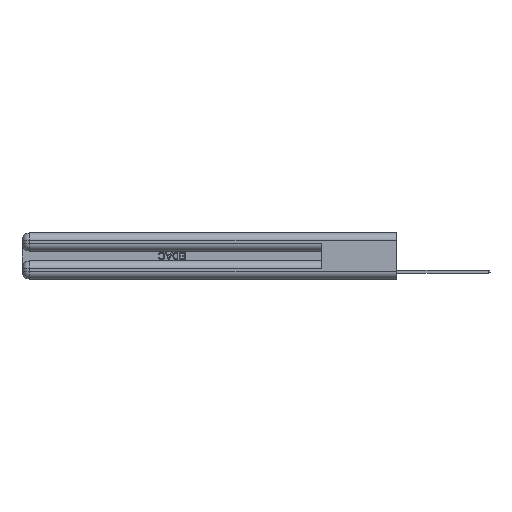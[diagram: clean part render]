
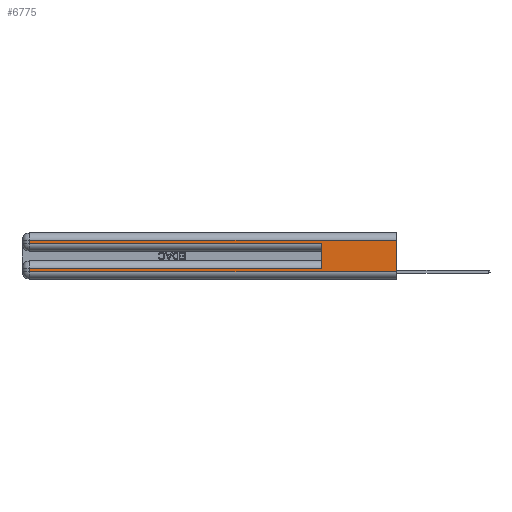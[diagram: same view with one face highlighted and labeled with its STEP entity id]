
A CAD part, left-side view. The second image highlights one B-rep face of the part: STEP entity #6775.
In plain terms, the highlighted planar face has unit normal (-1, 0, 0).
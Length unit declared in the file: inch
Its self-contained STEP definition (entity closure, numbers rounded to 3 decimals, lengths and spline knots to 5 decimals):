
#906 = EDGE_CURVE ( 'NONE', #27352, #23586, #1004, .T. ) ;
#1004 = LINE ( 'NONE', #22180, #7337 ) ;
#1892 = CARTESIAN_POINT ( 'NONE',  ( 0., 0.6, 0.085 ) ) ;
#3606 = VERTEX_POINT ( 'NONE', #33689 ) ;
#3704 = DIRECTION ( 'NONE',  ( 0., 0., 1. ) ) ;
#4698 = LINE ( 'NONE', #28986, #30235 ) ;
#5612 = DIRECTION ( 'NONE',  ( 0., 1., 0. ) ) ;
#5818 = CARTESIAN_POINT ( 'NONE',  ( 0., 0., 0.085 ) ) ;
#6775 = ADVANCED_FACE ( 'NONE', ( #32164 ), #9084, .F. ) ;
#7131 = EDGE_CURVE ( 'NONE', #3606, #16999, #32991, .T. ) ;
#7337 = VECTOR ( 'NONE', #27088, 39.37008 ) ;
#7918 = LINE ( 'NONE', #5818, #17480 ) ;
#9084 = PLANE ( 'NONE',  #31050 ) ;
#11957 = DIRECTION ( 'NONE',  ( 1., 0., 0. ) ) ;
#12300 = EDGE_CURVE ( 'NONE', #30285, #13682, #31809, .T. ) ;
#13682 = VERTEX_POINT ( 'NONE', #26045 ) ;
#13690 = CARTESIAN_POINT ( 'NONE',  ( 0., 0.6, 0.285 ) ) ;
#13974 = VERTEX_POINT ( 'NONE', #32302 ) ;
#14241 = CARTESIAN_POINT ( 'NONE',  ( 0., 0., 0.31 ) ) ;
#14755 = CARTESIAN_POINT ( 'NONE',  ( 0., 0., 0.37 ) ) ;
#15236 = CARTESIAN_POINT ( 'NONE',  ( 0., 2.94, 0.37 ) ) ;
#15735 = CARTESIAN_POINT ( 'NONE',  ( 0., 2.94, 0.06 ) ) ;
#16141 = EDGE_CURVE ( 'NONE', #16999, #13682, #31997, .T. ) ;
#16999 = VERTEX_POINT ( 'NONE', #15735 ) ;
#17001 = VERTEX_POINT ( 'NONE', #1892 ) ;
#17061 = DIRECTION ( 'NONE',  ( 0., 1., 0. ) ) ;
#17429 = DIRECTION ( 'NONE',  ( 0., 0., -1. ) ) ;
#17480 = VECTOR ( 'NONE', #17061, 39.37008 ) ;
#17542 = VECTOR ( 'NONE', #29058, 39.37008 ) ;
#17608 = EDGE_CURVE ( 'NONE', #13974, #27352, #4698, .T. ) ;
#17746 = CARTESIAN_POINT ( 'NONE',  ( 0., 0., 0.06 ) ) ;
#19185 = EDGE_CURVE ( 'NONE', #17001, #3606, #7918, .T. ) ;
#19552 = ORIENTED_EDGE ( 'NONE', *, *, #23334, .F. ) ;
#22180 = CARTESIAN_POINT ( 'NONE',  ( 0., 0., 0.285 ) ) ;
#22620 = ORIENTED_EDGE ( 'NONE', *, *, #17608, .T. ) ;
#22773 = EDGE_CURVE ( 'NONE', #30285, #13974, #31952, .T. ) ;
#22895 = VECTOR ( 'NONE', #22954, 39.37008 ) ;
#22954 = DIRECTION ( 'NONE',  ( 0., 0., -1. ) ) ;
#23334 = EDGE_CURVE ( 'NONE', #17001, #23586, #28950, .T. ) ;
#23498 = EDGE_LOOP ( 'NONE', ( #28323, #26094, #22620, #30544, #19552, #23530, #29161, #25673 ) ) ;
#23530 = ORIENTED_EDGE ( 'NONE', *, *, #19185, .T. ) ;
#23586 = VERTEX_POINT ( 'NONE', #13690 ) ;
#24133 = CARTESIAN_POINT ( 'NONE',  ( 0., 0., 0.31 ) ) ;
#25673 = ORIENTED_EDGE ( 'NONE', *, *, #16141, .T. ) ;
#25760 = CARTESIAN_POINT ( 'NONE',  ( 0., 0., 0.37 ) ) ;
#26020 = DIRECTION ( 'NONE',  ( 0., -1., 0. ) ) ;
#26045 = CARTESIAN_POINT ( 'NONE',  ( 0., 0., 0.06 ) ) ;
#26094 = ORIENTED_EDGE ( 'NONE', *, *, #22773, .T. ) ;
#26121 = DIRECTION ( 'NONE',  ( 0., 0., -1. ) ) ;
#27088 = DIRECTION ( 'NONE',  ( 0., -1., 0. ) ) ;
#27352 = VERTEX_POINT ( 'NONE', #31209 ) ;
#27699 = VECTOR ( 'NONE', #3704, 39.37008 ) ;
#28323 = ORIENTED_EDGE ( 'NONE', *, *, #12300, .F. ) ;
#28950 = LINE ( 'NONE', #32922, #27699 ) ;
#28986 = CARTESIAN_POINT ( 'NONE',  ( 0., 2.94, 0.37 ) ) ;
#29058 = DIRECTION ( 'NONE',  ( 0., 0., -1. ) ) ;
#29161 = ORIENTED_EDGE ( 'NONE', *, *, #7131, .T. ) ;
#30235 = VECTOR ( 'NONE', #26121, 39.37008 ) ;
#30285 = VERTEX_POINT ( 'NONE', #14241 ) ;
#30544 = ORIENTED_EDGE ( 'NONE', *, *, #906, .T. ) ;
#31050 = AXIS2_PLACEMENT_3D ( 'NONE', #14755, #11957, #17429 ) ;
#31209 = CARTESIAN_POINT ( 'NONE',  ( 0., 2.94, 0.285 ) ) ;
#31809 = LINE ( 'NONE', #25760, #17542 ) ;
#31952 = LINE ( 'NONE', #24133, #33663 ) ;
#31997 = LINE ( 'NONE', #17746, #33261 ) ;
#32164 = FACE_OUTER_BOUND ( 'NONE', #23498, .T. ) ;
#32302 = CARTESIAN_POINT ( 'NONE',  ( 0., 2.94, 0.31 ) ) ;
#32922 = CARTESIAN_POINT ( 'NONE',  ( 0., 0.6, 0.145 ) ) ;
#32991 = LINE ( 'NONE', #15236, #22895 ) ;
#33261 = VECTOR ( 'NONE', #26020, 39.37008 ) ;
#33663 = VECTOR ( 'NONE', #5612, 39.37008 ) ;
#33689 = CARTESIAN_POINT ( 'NONE',  ( 0., 2.94, 0.085 ) ) ;
